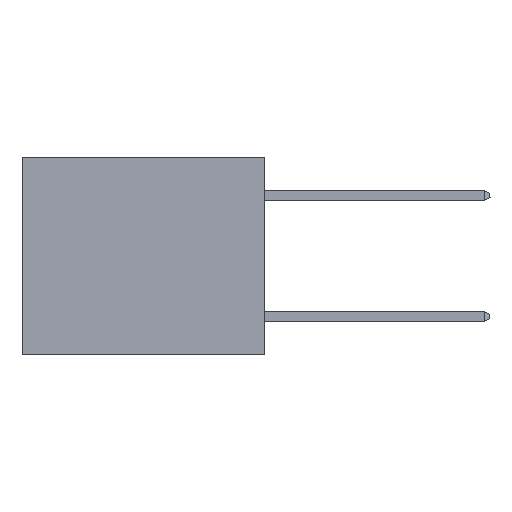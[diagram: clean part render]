
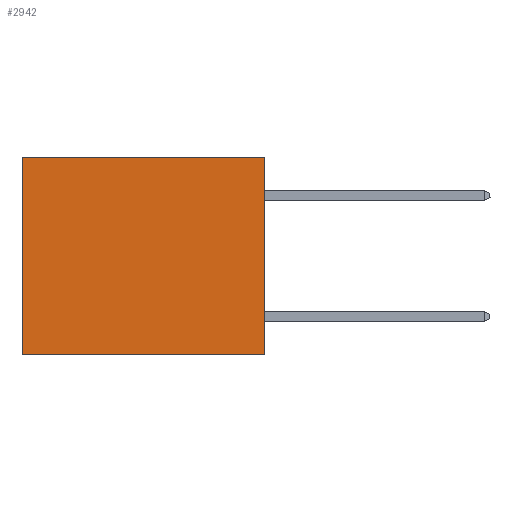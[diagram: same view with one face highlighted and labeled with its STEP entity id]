
A CAD part, left-side view. The second image highlights one B-rep face of the part: STEP entity #2942.
In plain terms, the highlighted planar face has unit normal (-1, 0, 0).
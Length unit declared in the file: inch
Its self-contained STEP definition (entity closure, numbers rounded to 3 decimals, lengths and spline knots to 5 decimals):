
#450 = EDGE_CURVE ( 'NONE', #20710, #2282, #17434, .T. ) ;
#2282 = VERTEX_POINT ( 'NONE', #7823 ) ;
#2367 = VECTOR ( 'NONE', #14491, 39.37008 ) ;
#2942 = ADVANCED_FACE ( 'NONE', ( #6700 ), #26504, .F. ) ;
#3365 = VECTOR ( 'NONE', #6623, 39.37008 ) ;
#5253 = ORIENTED_EDGE ( 'NONE', *, *, #27981, .F. ) ;
#5267 = ORIENTED_EDGE ( 'NONE', *, *, #16300, .T. ) ;
#6199 = CARTESIAN_POINT ( 'NONE',  ( 0.3165, 0.6, -0.49 ) ) ;
#6623 = DIRECTION ( 'NONE',  ( 0., 0., -1. ) ) ;
#6700 = FACE_OUTER_BOUND ( 'NONE', #17889, .T. ) ;
#6797 = EDGE_CURVE ( 'NONE', #17191, #2282, #16445, .T. ) ;
#7150 = VECTOR ( 'NONE', #10000, 39.37008 ) ;
#7579 = DIRECTION ( 'NONE',  ( 0., 0., -1. ) ) ;
#7823 = CARTESIAN_POINT ( 'NONE',  ( 0.3165, 0.6, -0.49 ) ) ;
#10000 = DIRECTION ( 'NONE',  ( 0., 0., -1. ) ) ;
#10896 = CARTESIAN_POINT ( 'NONE',  ( 0.3165, 0., 0. ) ) ;
#13872 = CARTESIAN_POINT ( 'NONE',  ( 0.3165, 0., 0. ) ) ;
#14162 = DIRECTION ( 'NONE',  ( 1., 0., 0. ) ) ;
#14315 = LINE ( 'NONE', #28221, #3365 ) ;
#14491 = DIRECTION ( 'NONE',  ( 0., 1., 0. ) ) ;
#16300 = EDGE_CURVE ( 'NONE', #26960, #20710, #20048, .T. ) ;
#16445 = LINE ( 'NONE', #18457, #2367 ) ;
#16924 = CARTESIAN_POINT ( 'NONE',  ( 0.3165, 0., -0.49 ) ) ;
#16960 = CARTESIAN_POINT ( 'NONE',  ( 0.3165, 0.6, 0. ) ) ;
#16994 = AXIS2_PLACEMENT_3D ( 'NONE', #22356, #14162, #7579 ) ;
#17191 = VERTEX_POINT ( 'NONE', #16924 ) ;
#17434 = LINE ( 'NONE', #6199, #7150 ) ;
#17889 = EDGE_LOOP ( 'NONE', ( #22451, #24743, #5253, #5267 ) ) ;
#18457 = CARTESIAN_POINT ( 'NONE',  ( 0.3165, 0., -0.49 ) ) ;
#20048 = LINE ( 'NONE', #10896, #23759 ) ;
#20710 = VERTEX_POINT ( 'NONE', #16960 ) ;
#22356 = CARTESIAN_POINT ( 'NONE',  ( 0.3165, 0., -0.49 ) ) ;
#22451 = ORIENTED_EDGE ( 'NONE', *, *, #450, .T. ) ;
#23759 = VECTOR ( 'NONE', #28212, 39.37008 ) ;
#24743 = ORIENTED_EDGE ( 'NONE', *, *, #6797, .F. ) ;
#26504 = PLANE ( 'NONE',  #16994 ) ;
#26960 = VERTEX_POINT ( 'NONE', #13872 ) ;
#27981 = EDGE_CURVE ( 'NONE', #26960, #17191, #14315, .T. ) ;
#28212 = DIRECTION ( 'NONE',  ( 0., 1., 0. ) ) ;
#28221 = CARTESIAN_POINT ( 'NONE',  ( 0.3165, 0., -0.49 ) ) ;
